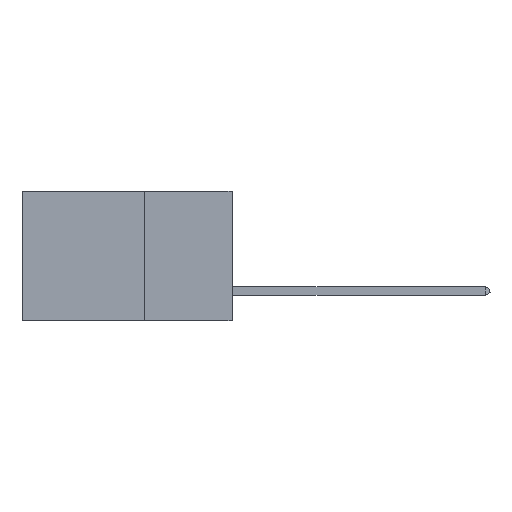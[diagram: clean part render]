
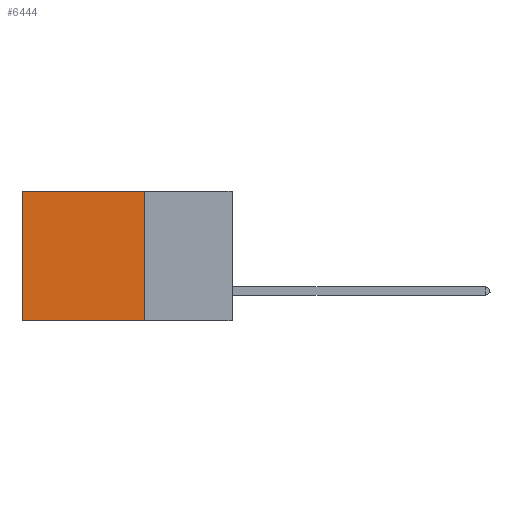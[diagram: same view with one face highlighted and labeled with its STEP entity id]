
A CAD part, left-side view. The second image highlights one B-rep face of the part: STEP entity #6444.
In plain terms, the highlighted planar face has unit normal (-1, 0, 0).
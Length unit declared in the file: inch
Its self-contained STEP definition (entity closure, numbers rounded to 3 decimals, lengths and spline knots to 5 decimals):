
#826 = CARTESIAN_POINT ( 'NONE',  ( 0.2875, 0.25, 0. ) ) ;
#1979 = PLANE ( 'NONE',  #19825 ) ;
#2499 = EDGE_CURVE ( 'NONE', #37368, #16063, #36943, .T. ) ;
#3422 = LINE ( 'NONE', #27076, #35557 ) ;
#6444 = ADVANCED_FACE ( 'NONE', ( #31759 ), #1979, .F. ) ;
#7716 = EDGE_CURVE ( 'NONE', #37368, #25459, #3422, .T. ) ;
#8266 = CARTESIAN_POINT ( 'NONE',  ( 0.2875, 0.6, 0. ) ) ;
#8993 = DIRECTION ( 'NONE',  ( 0., 1., 0. ) ) ;
#9741 = CARTESIAN_POINT ( 'NONE',  ( 0.2875, 0.25, -0.37 ) ) ;
#10783 = DIRECTION ( 'NONE',  ( 1., 0., 0. ) ) ;
#11076 = DIRECTION ( 'NONE',  ( 0., 0., -1. ) ) ;
#11380 = VECTOR ( 'NONE', #8993, 39.37008 ) ;
#14124 = ORIENTED_EDGE ( 'NONE', *, *, #7716, .T. ) ;
#16063 = VERTEX_POINT ( 'NONE', #9741 ) ;
#17558 = EDGE_CURVE ( 'NONE', #16063, #24004, #26450, .T. ) ;
#18639 = EDGE_LOOP ( 'NONE', ( #37382, #29385, #19804, #14124 ) ) ;
#19804 = ORIENTED_EDGE ( 'NONE', *, *, #2499, .F. ) ;
#19825 = AXIS2_PLACEMENT_3D ( 'NONE', #29450, #10783, #20016 ) ;
#20016 = DIRECTION ( 'NONE',  ( 0., 0., -1. ) ) ;
#20330 = VECTOR ( 'NONE', #11076, 39.37008 ) ;
#20738 = DIRECTION ( 'NONE',  ( 0., 0., -1. ) ) ;
#23862 = LINE ( 'NONE', #8266, #32106 ) ;
#24004 = VERTEX_POINT ( 'NONE', #37205 ) ;
#24535 = EDGE_CURVE ( 'NONE', #25459, #24004, #23862, .T. ) ;
#25459 = VERTEX_POINT ( 'NONE', #31571 ) ;
#26450 = LINE ( 'NONE', #39901, #11380 ) ;
#27076 = CARTESIAN_POINT ( 'NONE',  ( 0.2875, 0.25, 0. ) ) ;
#29385 = ORIENTED_EDGE ( 'NONE', *, *, #17558, .F. ) ;
#29450 = CARTESIAN_POINT ( 'NONE',  ( 0.2875, 0.25, 0. ) ) ;
#31571 = CARTESIAN_POINT ( 'NONE',  ( 0.2875, 0.6, 0. ) ) ;
#31759 = FACE_OUTER_BOUND ( 'NONE', #18639, .T. ) ;
#32106 = VECTOR ( 'NONE', #20738, 39.37008 ) ;
#33998 = CARTESIAN_POINT ( 'NONE',  ( 0.2875, 0.25, 0. ) ) ;
#35557 = VECTOR ( 'NONE', #39619, 39.37008 ) ;
#36943 = LINE ( 'NONE', #33998, #20330 ) ;
#37205 = CARTESIAN_POINT ( 'NONE',  ( 0.2875, 0.6, -0.37 ) ) ;
#37368 = VERTEX_POINT ( 'NONE', #826 ) ;
#37382 = ORIENTED_EDGE ( 'NONE', *, *, #24535, .T. ) ;
#39619 = DIRECTION ( 'NONE',  ( 0., 1., 0. ) ) ;
#39901 = CARTESIAN_POINT ( 'NONE',  ( 0.2875, 0.25, -0.37 ) ) ;
